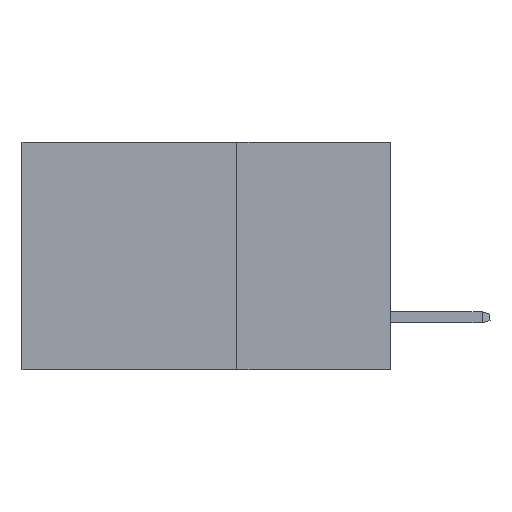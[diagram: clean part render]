
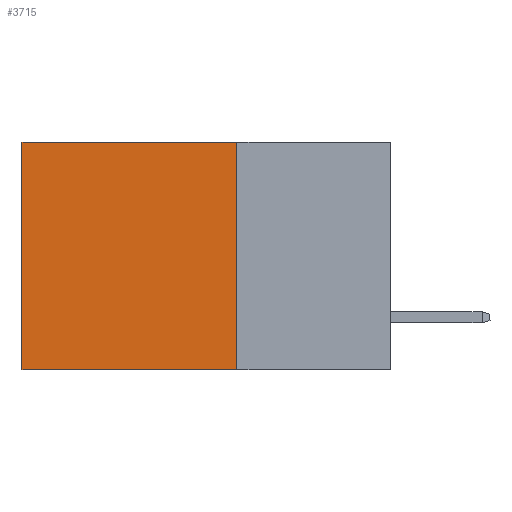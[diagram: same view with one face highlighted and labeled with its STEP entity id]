
A CAD part, left-side view. The second image highlights one B-rep face of the part: STEP entity #3715.
In plain terms, the highlighted planar face has unit normal (-1, 0, 0).
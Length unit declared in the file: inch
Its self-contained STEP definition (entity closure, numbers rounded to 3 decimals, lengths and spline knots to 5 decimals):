
#115 = LINE ( 'NONE', #28186, #17376 ) ;
#1204 = DIRECTION ( 'NONE',  ( 0., 0., -1. ) ) ;
#1386 = DIRECTION ( 'NONE',  ( 0., 1., 0. ) ) ;
#1816 = CARTESIAN_POINT ( 'NONE',  ( 0.2875, 0.25, 0. ) ) ;
#1955 = CARTESIAN_POINT ( 'NONE',  ( 0.2875, 0.6, -0.37 ) ) ;
#2904 = ORIENTED_EDGE ( 'NONE', *, *, #25640, .F. ) ;
#3715 = ADVANCED_FACE ( 'NONE', ( #15866 ), #15739, .F. ) ;
#4514 = DIRECTION ( 'NONE',  ( 1., 0., 0. ) ) ;
#5282 = CARTESIAN_POINT ( 'NONE',  ( 0.2875, 0.25, 0. ) ) ;
#6257 = CARTESIAN_POINT ( 'NONE',  ( 0.2875, 0.25, -0.37 ) ) ;
#7708 = VECTOR ( 'NONE', #28435, 39.37008 ) ;
#7937 = VECTOR ( 'NONE', #1386, 39.37008 ) ;
#8185 = EDGE_LOOP ( 'NONE', ( #8272, #18130, #2904, #23879 ) ) ;
#8272 = ORIENTED_EDGE ( 'NONE', *, *, #10910, .T. ) ;
#10910 = EDGE_CURVE ( 'NONE', #22779, #27553, #115, .T. ) ;
#13912 = LINE ( 'NONE', #19290, #7937 ) ;
#14378 = VERTEX_POINT ( 'NONE', #6257 ) ;
#14984 = CARTESIAN_POINT ( 'NONE',  ( 0.2875, 0.25, 0. ) ) ;
#15739 = PLANE ( 'NONE',  #26920 ) ;
#15866 = FACE_OUTER_BOUND ( 'NONE', #8185, .T. ) ;
#17376 = VECTOR ( 'NONE', #1204, 39.37008 ) ;
#17567 = DIRECTION ( 'NONE',  ( 0., 0., -1. ) ) ;
#17989 = CARTESIAN_POINT ( 'NONE',  ( 0.2875, 0.25, 0. ) ) ;
#18130 = ORIENTED_EDGE ( 'NONE', *, *, #27369, .F. ) ;
#19290 = CARTESIAN_POINT ( 'NONE',  ( 0.2875, 0.25, -0.37 ) ) ;
#20224 = DIRECTION ( 'NONE',  ( 0., 0., -1. ) ) ;
#20256 = LINE ( 'NONE', #1816, #25563 ) ;
#22538 = CARTESIAN_POINT ( 'NONE',  ( 0.2875, 0.6, 0. ) ) ;
#22779 = VERTEX_POINT ( 'NONE', #22538 ) ;
#23879 = ORIENTED_EDGE ( 'NONE', *, *, #24836, .T. ) ;
#24836 = EDGE_CURVE ( 'NONE', #28500, #22779, #24894, .T. ) ;
#24894 = LINE ( 'NONE', #14984, #7708 ) ;
#25563 = VECTOR ( 'NONE', #17567, 39.37008 ) ;
#25640 = EDGE_CURVE ( 'NONE', #28500, #14378, #20256, .T. ) ;
#26920 = AXIS2_PLACEMENT_3D ( 'NONE', #17989, #4514, #20224 ) ;
#27369 = EDGE_CURVE ( 'NONE', #14378, #27553, #13912, .T. ) ;
#27553 = VERTEX_POINT ( 'NONE', #1955 ) ;
#28186 = CARTESIAN_POINT ( 'NONE',  ( 0.2875, 0.6, 0. ) ) ;
#28435 = DIRECTION ( 'NONE',  ( 0., 1., 0. ) ) ;
#28500 = VERTEX_POINT ( 'NONE', #5282 ) ;
